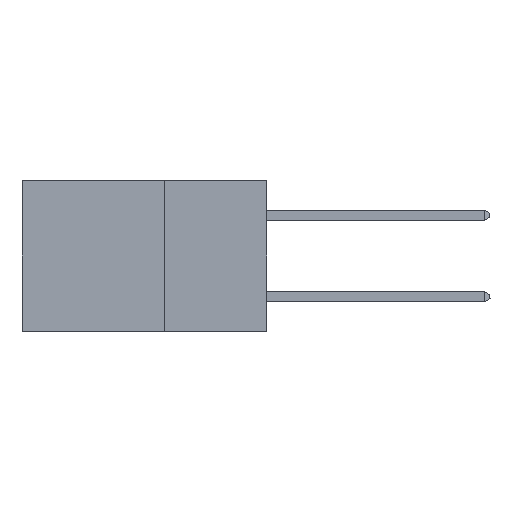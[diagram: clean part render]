
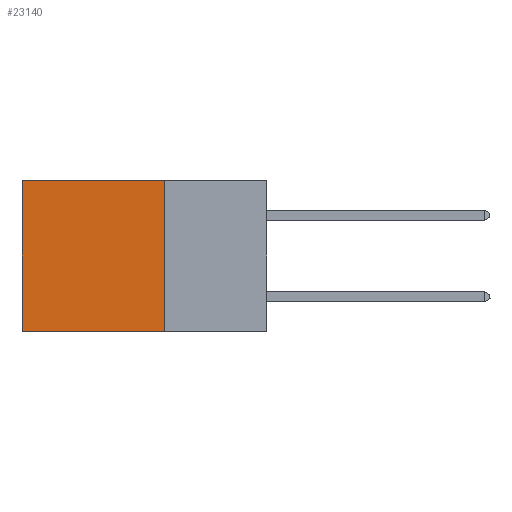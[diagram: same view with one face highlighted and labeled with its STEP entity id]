
A CAD part, left-side view. The second image highlights one B-rep face of the part: STEP entity #23140.
In plain terms, the highlighted planar face has unit normal (-1, 0, 0).
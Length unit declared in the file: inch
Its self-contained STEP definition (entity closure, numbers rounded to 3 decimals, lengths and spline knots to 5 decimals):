
#609 = VERTEX_POINT ( 'NONE', #13418 ) ;
#802 = DIRECTION ( 'NONE',  ( 0., 0., -1. ) ) ;
#1638 = CARTESIAN_POINT ( 'NONE',  ( 0.2875, 0.6, 0. ) ) ;
#1981 = VECTOR ( 'NONE', #16741, 39.37008 ) ;
#2033 = CARTESIAN_POINT ( 'NONE',  ( 0.2875, 0.25, 0. ) ) ;
#3630 = DIRECTION ( 'NONE',  ( 0., 1., 0. ) ) ;
#4585 = EDGE_CURVE ( 'NONE', #609, #15948, #5349, .T. ) ;
#4799 = EDGE_CURVE ( 'NONE', #15948, #22302, #13135, .T. ) ;
#5302 = EDGE_CURVE ( 'NONE', #609, #5335, #19854, .T. ) ;
#5335 = VERTEX_POINT ( 'NONE', #1638 ) ;
#5349 = LINE ( 'NONE', #13464, #7489 ) ;
#6384 = VECTOR ( 'NONE', #802, 39.37008 ) ;
#6400 = ORIENTED_EDGE ( 'NONE', *, *, #5302, .T. ) ;
#7489 = VECTOR ( 'NONE', #15472, 39.37008 ) ;
#8640 = AXIS2_PLACEMENT_3D ( 'NONE', #18507, #22235, #16245 ) ;
#9104 = ORIENTED_EDGE ( 'NONE', *, *, #4799, .F. ) ;
#9815 = CARTESIAN_POINT ( 'NONE',  ( 0.2875, 0.6, -0.37 ) ) ;
#10142 = EDGE_LOOP ( 'NONE', ( #16664, #9104, #15141, #6400 ) ) ;
#10904 = VECTOR ( 'NONE', #3630, 39.37008 ) ;
#11618 = EDGE_CURVE ( 'NONE', #5335, #22302, #16888, .T. ) ;
#13135 = LINE ( 'NONE', #25395, #1981 ) ;
#13418 = CARTESIAN_POINT ( 'NONE',  ( 0.2875, 0.25, 0. ) ) ;
#13464 = CARTESIAN_POINT ( 'NONE',  ( 0.2875, 0.25, 0. ) ) ;
#14642 = PLANE ( 'NONE',  #8640 ) ;
#15141 = ORIENTED_EDGE ( 'NONE', *, *, #4585, .F. ) ;
#15472 = DIRECTION ( 'NONE',  ( 0., 0., -1. ) ) ;
#15734 = CARTESIAN_POINT ( 'NONE',  ( 0.2875, 0.25, -0.37 ) ) ;
#15948 = VERTEX_POINT ( 'NONE', #15734 ) ;
#16245 = DIRECTION ( 'NONE',  ( 0., 0., -1. ) ) ;
#16631 = FACE_OUTER_BOUND ( 'NONE', #10142, .T. ) ;
#16664 = ORIENTED_EDGE ( 'NONE', *, *, #11618, .T. ) ;
#16741 = DIRECTION ( 'NONE',  ( 0., 1., 0. ) ) ;
#16888 = LINE ( 'NONE', #25289, #6384 ) ;
#18507 = CARTESIAN_POINT ( 'NONE',  ( 0.2875, 0.25, 0. ) ) ;
#19854 = LINE ( 'NONE', #2033, #10904 ) ;
#22235 = DIRECTION ( 'NONE',  ( 1., 0., 0. ) ) ;
#22302 = VERTEX_POINT ( 'NONE', #9815 ) ;
#23140 = ADVANCED_FACE ( 'NONE', ( #16631 ), #14642, .F. ) ;
#25289 = CARTESIAN_POINT ( 'NONE',  ( 0.2875, 0.6, 0. ) ) ;
#25395 = CARTESIAN_POINT ( 'NONE',  ( 0.2875, 0.25, -0.37 ) ) ;
